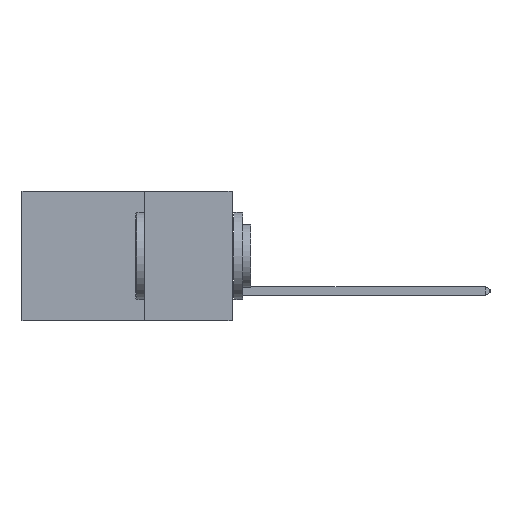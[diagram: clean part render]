
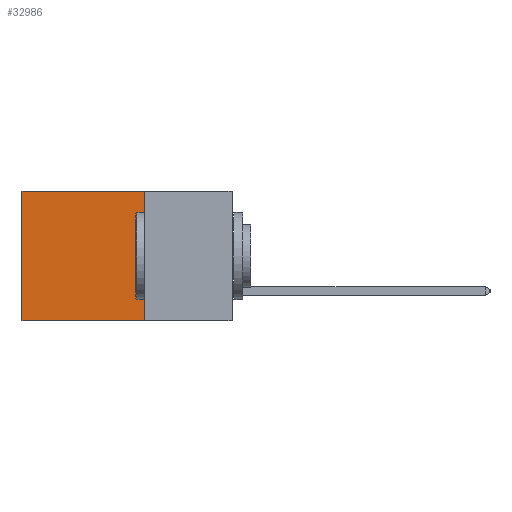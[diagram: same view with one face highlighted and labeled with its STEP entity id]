
A CAD part, left-side view. The second image highlights one B-rep face of the part: STEP entity #32986.
In plain terms, the highlighted planar face has unit normal (-1, 0, 0).
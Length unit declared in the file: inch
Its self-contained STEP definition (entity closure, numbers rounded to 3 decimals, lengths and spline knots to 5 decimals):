
#3656 = EDGE_CURVE ( 'NONE', #18252, #25874, #9260, .T. ) ;
#4364 = CARTESIAN_POINT ( 'NONE',  ( 0.2875, 0.6, 0. ) ) ;
#7295 = EDGE_CURVE ( 'NONE', #25874, #7501, #29036, .T. ) ;
#7501 = VERTEX_POINT ( 'NONE', #14632 ) ;
#7839 = ORIENTED_EDGE ( 'NONE', *, *, #19180, .T. ) ;
#8136 = EDGE_LOOP ( 'NONE', ( #11422, #37403, #41962, #7839 ) ) ;
#9124 = DIRECTION ( 'NONE',  ( 0., 1., 0. ) ) ;
#9260 = LINE ( 'NONE', #35534, #34479 ) ;
#11422 = ORIENTED_EDGE ( 'NONE', *, *, #21123, .T. ) ;
#12891 = PLANE ( 'NONE',  #40984 ) ;
#14632 = CARTESIAN_POINT ( 'NONE',  ( 0.2875, 0.6, -0.37 ) ) ;
#15137 = VERTEX_POINT ( 'NONE', #4364 ) ;
#15639 = DIRECTION ( 'NONE',  ( 0., 1., 0. ) ) ;
#15842 = CARTESIAN_POINT ( 'NONE',  ( 0.2875, 0.25, 0. ) ) ;
#18252 = VERTEX_POINT ( 'NONE', #15842 ) ;
#19180 = EDGE_CURVE ( 'NONE', #18252, #15137, #40114, .T. ) ;
#20548 = FACE_OUTER_BOUND ( 'NONE', #8136, .T. ) ;
#21123 = EDGE_CURVE ( 'NONE', #15137, #7501, #41296, .T. ) ;
#22276 = VECTOR ( 'NONE', #35953, 39.37008 ) ;
#23856 = VECTOR ( 'NONE', #15639, 39.37008 ) ;
#25697 = CARTESIAN_POINT ( 'NONE',  ( 0.2875, 0.25, 0. ) ) ;
#25874 = VERTEX_POINT ( 'NONE', #39162 ) ;
#26009 = DIRECTION ( 'NONE',  ( 0., 0., -1. ) ) ;
#26123 = DIRECTION ( 'NONE',  ( 1., 0., 0. ) ) ;
#28455 = CARTESIAN_POINT ( 'NONE',  ( 0.2875, 0.25, -0.37 ) ) ;
#29036 = LINE ( 'NONE', #28455, #23856 ) ;
#29477 = CARTESIAN_POINT ( 'NONE',  ( 0.2875, 0.6, 0. ) ) ;
#31417 = VECTOR ( 'NONE', #9124, 39.37008 ) ;
#32986 = ADVANCED_FACE ( 'NONE', ( #20548 ), #12891, .F. ) ;
#34479 = VECTOR ( 'NONE', #26009, 39.37008 ) ;
#35534 = CARTESIAN_POINT ( 'NONE',  ( 0.2875, 0.25, 0. ) ) ;
#35915 = DIRECTION ( 'NONE',  ( 0., 0., -1. ) ) ;
#35953 = DIRECTION ( 'NONE',  ( 0., 0., -1. ) ) ;
#37403 = ORIENTED_EDGE ( 'NONE', *, *, #7295, .F. ) ;
#38460 = CARTESIAN_POINT ( 'NONE',  ( 0.2875, 0.25, 0. ) ) ;
#39162 = CARTESIAN_POINT ( 'NONE',  ( 0.2875, 0.25, -0.37 ) ) ;
#40114 = LINE ( 'NONE', #38460, #31417 ) ;
#40984 = AXIS2_PLACEMENT_3D ( 'NONE', #25697, #26123, #35915 ) ;
#41296 = LINE ( 'NONE', #29477, #22276 ) ;
#41962 = ORIENTED_EDGE ( 'NONE', *, *, #3656, .F. ) ;
